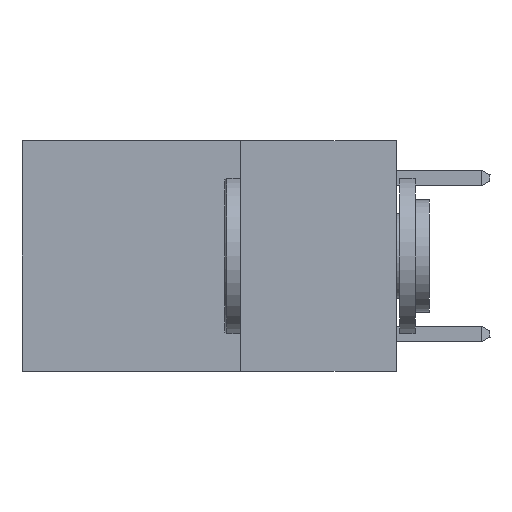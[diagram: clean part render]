
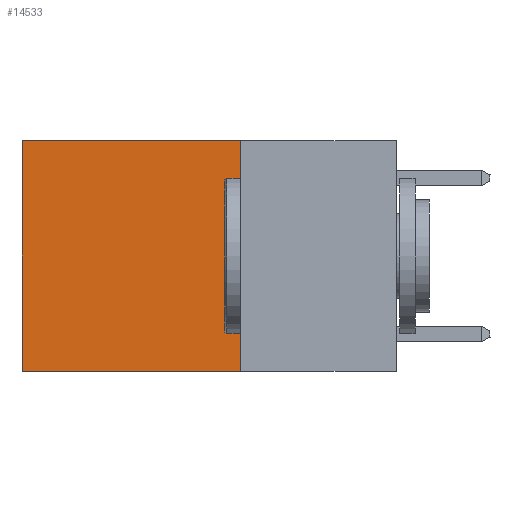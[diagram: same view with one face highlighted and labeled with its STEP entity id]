
A CAD part, left-side view. The second image highlights one B-rep face of the part: STEP entity #14533.
In plain terms, the highlighted planar face has unit normal (-1, 0, 0).
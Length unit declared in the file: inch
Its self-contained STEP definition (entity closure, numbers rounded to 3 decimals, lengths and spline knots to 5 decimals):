
#465 = VERTEX_POINT ( 'NONE', #13088 ) ;
#521 = ORIENTED_EDGE ( 'NONE', *, *, #16556, .T. ) ;
#1108 = ORIENTED_EDGE ( 'NONE', *, *, #3151, .T. ) ;
#1260 = CARTESIAN_POINT ( 'NONE',  ( 0.2625, 0.25, -0.37 ) ) ;
#1977 = CARTESIAN_POINT ( 'NONE',  ( 0.2625, 0.25, -0.37 ) ) ;
#2534 = DIRECTION ( 'NONE',  ( 0., 0., -1. ) ) ;
#2797 = LINE ( 'NONE', #1260, #8298 ) ;
#3030 = CARTESIAN_POINT ( 'NONE',  ( 0.2625, 0.25, 0. ) ) ;
#3151 = EDGE_CURVE ( 'NONE', #3757, #465, #9237, .T. ) ;
#3329 = VECTOR ( 'NONE', #15840, 39.37008 ) ;
#3757 = VERTEX_POINT ( 'NONE', #13468 ) ;
#4136 = CARTESIAN_POINT ( 'NONE',  ( 0.2625, 0.25, 0. ) ) ;
#4551 = CARTESIAN_POINT ( 'NONE',  ( 0.2625, 0.25, 0. ) ) ;
#5876 = VERTEX_POINT ( 'NONE', #1977 ) ;
#5954 = ORIENTED_EDGE ( 'NONE', *, *, #16068, .F. ) ;
#6690 = DIRECTION ( 'NONE',  ( 0., 0., -1. ) ) ;
#7049 = VECTOR ( 'NONE', #9365, 39.37008 ) ;
#7293 = AXIS2_PLACEMENT_3D ( 'NONE', #4136, #7827, #2534 ) ;
#7413 = VECTOR ( 'NONE', #6690, 39.37008 ) ;
#7827 = DIRECTION ( 'NONE',  ( 1., 0., 0. ) ) ;
#7957 = CARTESIAN_POINT ( 'NONE',  ( 0.2625, 0.6, 0. ) ) ;
#7989 = EDGE_CURVE ( 'NONE', #5876, #465, #2797, .T. ) ;
#8298 = VECTOR ( 'NONE', #9037, 39.37008 ) ;
#9037 = DIRECTION ( 'NONE',  ( 0., 1., 0. ) ) ;
#9237 = LINE ( 'NONE', #7957, #7413 ) ;
#9365 = DIRECTION ( 'NONE',  ( 0., 0., -1. ) ) ;
#9590 = ORIENTED_EDGE ( 'NONE', *, *, #7989, .F. ) ;
#10704 = LINE ( 'NONE', #15698, #7049 ) ;
#11690 = VERTEX_POINT ( 'NONE', #4551 ) ;
#11893 = EDGE_LOOP ( 'NONE', ( #1108, #9590, #5954, #521 ) ) ;
#12695 = PLANE ( 'NONE',  #7293 ) ;
#13088 = CARTESIAN_POINT ( 'NONE',  ( 0.2625, 0.6, -0.37 ) ) ;
#13468 = CARTESIAN_POINT ( 'NONE',  ( 0.2625, 0.6, 0. ) ) ;
#14533 = ADVANCED_FACE ( 'NONE', ( #15367 ), #12695, .F. ) ;
#15367 = FACE_OUTER_BOUND ( 'NONE', #11893, .T. ) ;
#15698 = CARTESIAN_POINT ( 'NONE',  ( 0.2625, 0.25, 0. ) ) ;
#15840 = DIRECTION ( 'NONE',  ( 0., 1., 0. ) ) ;
#16015 = LINE ( 'NONE', #3030, #3329 ) ;
#16068 = EDGE_CURVE ( 'NONE', #11690, #5876, #10704, .T. ) ;
#16556 = EDGE_CURVE ( 'NONE', #11690, #3757, #16015, .T. ) ;
